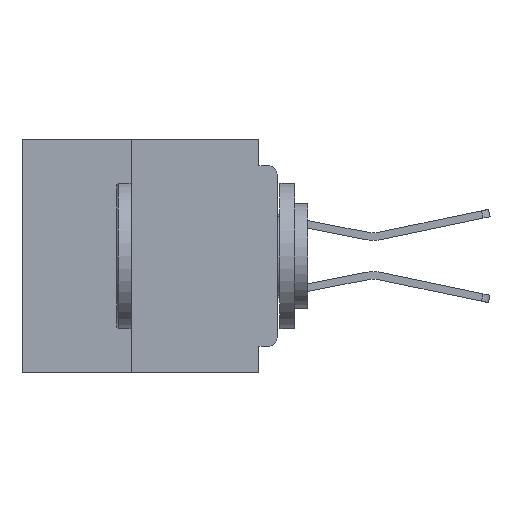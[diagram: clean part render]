
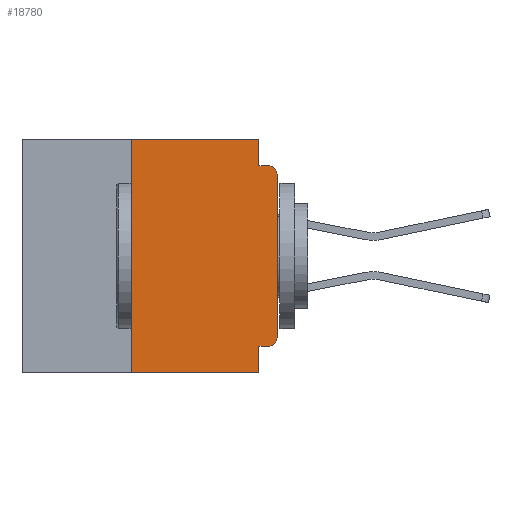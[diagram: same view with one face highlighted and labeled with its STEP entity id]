
A CAD part, left-side view. The second image highlights one B-rep face of the part: STEP entity #18780.
In plain terms, the highlighted planar face has unit normal (-1, 0, 0).
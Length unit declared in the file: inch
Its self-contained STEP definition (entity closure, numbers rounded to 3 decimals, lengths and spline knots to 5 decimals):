
#69 = VERTEX_POINT ( 'NONE', #54322 ) ;
#2105 = AXIS2_PLACEMENT_3D ( 'NONE', #19210, #51292, #23807 ) ;
#2159 = CARTESIAN_POINT ( 'NONE',  ( 0., 0.437, 0. ) ) ;
#2502 = DIRECTION ( 'NONE',  ( 0., 1., 0. ) ) ;
#2690 = VECTOR ( 'NONE', #2502, 39.37008 ) ;
#4370 = CIRCLE ( 'NONE', #44550, 0.015 ) ;
#4942 = CARTESIAN_POINT ( 'NONE',  ( 0., 0.015, -0.355 ) ) ;
#5082 = CARTESIAN_POINT ( 'NONE',  ( 0., 0., 0. ) ) ;
#6343 = AXIS2_PLACEMENT_3D ( 'NONE', #2159, #20767, #52827 ) ;
#7611 = DIRECTION ( 'NONE',  ( 0., 0., -1. ) ) ;
#8518 = LINE ( 'NONE', #47754, #19376 ) ;
#8651 = EDGE_CURVE ( 'NONE', #35854, #36263, #16499, .T. ) ;
#8951 = EDGE_CURVE ( 'NONE', #15738, #69, #37213, .T. ) ;
#10803 = ORIENTED_EDGE ( 'NONE', *, *, #8951, .F. ) ;
#11149 = ORIENTED_EDGE ( 'NONE', *, *, #23547, .F. ) ;
#13325 = EDGE_CURVE ( 'NONE', #38287, #15738, #52252, .T. ) ;
#14043 = DIRECTION ( 'NONE',  ( 0., -1., 0. ) ) ;
#14715 = EDGE_LOOP ( 'NONE', ( #44658, #21983, #10803, #55702, #19309, #22521, #42775, #40547, #11149, #37932 ) ) ;
#15738 = VERTEX_POINT ( 'NONE', #54269 ) ;
#16122 = PLANE ( 'NONE',  #6343 ) ;
#16499 = LINE ( 'NONE', #41510, #17947 ) ;
#17216 = CARTESIAN_POINT ( 'NONE',  ( 0., 0.031, 0. ) ) ;
#17413 = VERTEX_POINT ( 'NONE', #4942 ) ;
#17947 = VECTOR ( 'NONE', #14043, 39.37008 ) ;
#18780 = ADVANCED_FACE ( 'NONE', ( #45035 ), #16122, .F. ) ;
#19210 = CARTESIAN_POINT ( 'NONE',  ( 0., 0.015, -0.06 ) ) ;
#19309 = ORIENTED_EDGE ( 'NONE', *, *, #23475, .F. ) ;
#19376 = VECTOR ( 'NONE', #52366, 39.37008 ) ;
#20767 = DIRECTION ( 'NONE',  ( 1., 0., 0. ) ) ;
#20781 = CARTESIAN_POINT ( 'NONE',  ( 0., 0.015, -0.34 ) ) ;
#20817 = LINE ( 'NONE', #52503, #55954 ) ;
#20872 = DIRECTION ( 'NONE',  ( 0., -1., 0. ) ) ;
#21842 = DIRECTION ( 'NONE',  ( 0., 0., -1. ) ) ;
#21983 = ORIENTED_EDGE ( 'NONE', *, *, #38771, .T. ) ;
#22521 = ORIENTED_EDGE ( 'NONE', *, *, #52367, .F. ) ;
#22545 = LINE ( 'NONE', #5082, #45445 ) ;
#23475 = EDGE_CURVE ( 'NONE', #51732, #38287, #8518, .T. ) ;
#23547 = EDGE_CURVE ( 'NONE', #17413, #37986, #51631, .T. ) ;
#23807 = DIRECTION ( 'NONE',  ( 0., 0., -1. ) ) ;
#25042 = VECTOR ( 'NONE', #20872, 39.37008 ) ;
#25340 = DIRECTION ( 'NONE',  ( 0., 0., -1. ) ) ;
#25779 = CARTESIAN_POINT ( 'NONE',  ( 0., 0.031, -0.4 ) ) ;
#27526 = CARTESIAN_POINT ( 'NONE',  ( 0., 0.031, -0.355 ) ) ;
#27871 = VECTOR ( 'NONE', #21842, 39.37008 ) ;
#27970 = CIRCLE ( 'NONE', #2105, 0.015 ) ;
#28085 = DIRECTION ( 'NONE',  ( 0., 0., 1. ) ) ;
#29433 = VERTEX_POINT ( 'NONE', #33338 ) ;
#29634 = DIRECTION ( 'NONE',  ( 0., 0., 1. ) ) ;
#30512 = EDGE_CURVE ( 'NONE', #29433, #57029, #22545, .T. ) ;
#33338 = CARTESIAN_POINT ( 'NONE',  ( 0., 0., -0.34 ) ) ;
#35123 = CARTESIAN_POINT ( 'NONE',  ( 0., 0.031, -0.4 ) ) ;
#35854 = VERTEX_POINT ( 'NONE', #40840 ) ;
#36263 = VERTEX_POINT ( 'NONE', #25779 ) ;
#37213 = LINE ( 'NONE', #48321, #25042 ) ;
#37932 = ORIENTED_EDGE ( 'NONE', *, *, #50830, .T. ) ;
#37986 = VERTEX_POINT ( 'NONE', #27526 ) ;
#38287 = VERTEX_POINT ( 'NONE', #52517 ) ;
#38771 = EDGE_CURVE ( 'NONE', #57029, #69, #27970, .T. ) ;
#40547 = ORIENTED_EDGE ( 'NONE', *, *, #46293, .F. ) ;
#40560 = LINE ( 'NONE', #35123, #51388 ) ;
#40840 = CARTESIAN_POINT ( 'NONE',  ( 0., 0.25, -0.4 ) ) ;
#41510 = CARTESIAN_POINT ( 'NONE',  ( 0., 0.437, -0.4 ) ) ;
#42775 = ORIENTED_EDGE ( 'NONE', *, *, #8651, .T. ) ;
#44550 = AXIS2_PLACEMENT_3D ( 'NONE', #20781, #52838, #25340 ) ;
#44658 = ORIENTED_EDGE ( 'NONE', *, *, #30512, .T. ) ;
#45035 = FACE_OUTER_BOUND ( 'NONE', #14715, .T. ) ;
#45445 = VECTOR ( 'NONE', #28085, 39.37008 ) ;
#46293 = EDGE_CURVE ( 'NONE', #37986, #36263, #40560, .T. ) ;
#47754 = CARTESIAN_POINT ( 'NONE',  ( 0., 0.437, 0. ) ) ;
#48172 = CARTESIAN_POINT ( 'NONE',  ( 0., 0.25, 0. ) ) ;
#48321 = CARTESIAN_POINT ( 'NONE',  ( 0., 0., -0.045 ) ) ;
#48358 = CARTESIAN_POINT ( 'NONE',  ( 0., 0., -0.355 ) ) ;
#50830 = EDGE_CURVE ( 'NONE', #17413, #29433, #4370, .T. ) ;
#51292 = DIRECTION ( 'NONE',  ( -1., 0., 0. ) ) ;
#51388 = VECTOR ( 'NONE', #7611, 39.37008 ) ;
#51631 = LINE ( 'NONE', #48358, #2690 ) ;
#51732 = VERTEX_POINT ( 'NONE', #48172 ) ;
#52252 = LINE ( 'NONE', #17216, #27871 ) ;
#52366 = DIRECTION ( 'NONE',  ( 0., -1., 0. ) ) ;
#52367 = EDGE_CURVE ( 'NONE', #35854, #51732, #20817, .T. ) ;
#52503 = CARTESIAN_POINT ( 'NONE',  ( 0., 0.25, -0.4 ) ) ;
#52517 = CARTESIAN_POINT ( 'NONE',  ( 0., 0.031, 0. ) ) ;
#52827 = DIRECTION ( 'NONE',  ( 0., 0., -1. ) ) ;
#52838 = DIRECTION ( 'NONE',  ( -1., 0., 0. ) ) ;
#54269 = CARTESIAN_POINT ( 'NONE',  ( 0., 0.031, -0.045 ) ) ;
#54322 = CARTESIAN_POINT ( 'NONE',  ( 0., 0.015, -0.045 ) ) ;
#55702 = ORIENTED_EDGE ( 'NONE', *, *, #13325, .F. ) ;
#55954 = VECTOR ( 'NONE', #29634, 39.37008 ) ;
#56008 = CARTESIAN_POINT ( 'NONE',  ( 0., 0., -0.06 ) ) ;
#57029 = VERTEX_POINT ( 'NONE', #56008 ) ;
